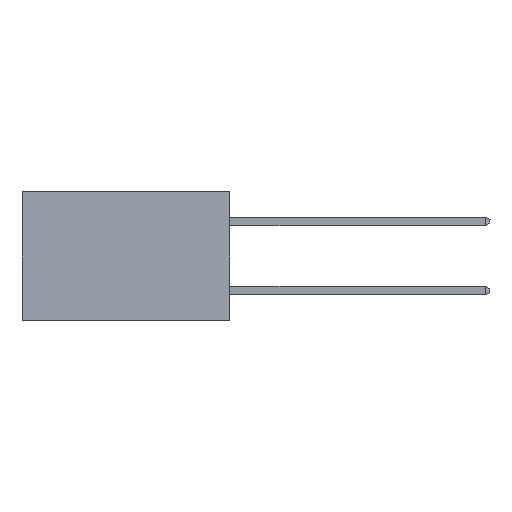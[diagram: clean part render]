
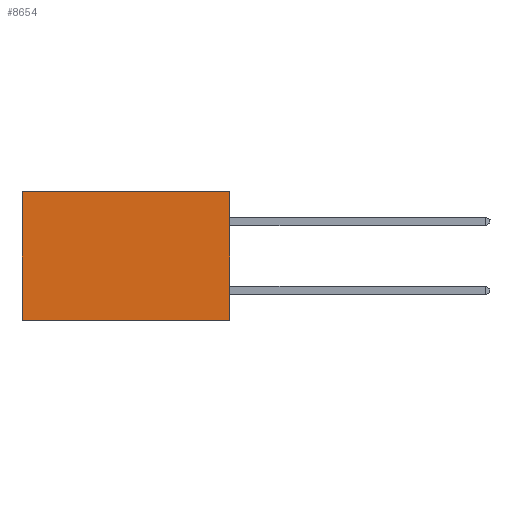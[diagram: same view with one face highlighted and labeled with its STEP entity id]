
A CAD part, left-side view. The second image highlights one B-rep face of the part: STEP entity #8654.
In plain terms, the highlighted planar face has unit normal (-1, 0, 0).
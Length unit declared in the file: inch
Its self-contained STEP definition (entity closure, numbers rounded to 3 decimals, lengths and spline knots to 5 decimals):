
#63 = EDGE_CURVE ( 'NONE', #13711, #1478, #19436, .T. ) ;
#925 = DIRECTION ( 'NONE',  ( 0., 0., -1. ) ) ;
#1478 = VERTEX_POINT ( 'NONE', #13507 ) ;
#2407 = DIRECTION ( 'NONE',  ( 0., 1., 0. ) ) ;
#2494 = ORIENTED_EDGE ( 'NONE', *, *, #6454, .F. ) ;
#3353 = VECTOR ( 'NONE', #8710, 39.37008 ) ;
#4126 = VECTOR ( 'NONE', #11520, 39.37008 ) ;
#4260 = VECTOR ( 'NONE', #9611, 39.37008 ) ;
#4748 = LINE ( 'NONE', #16527, #4126 ) ;
#5130 = VECTOR ( 'NONE', #2407, 39.37008 ) ;
#5297 = EDGE_CURVE ( 'NONE', #5812, #1478, #11095, .T. ) ;
#5747 = ORIENTED_EDGE ( 'NONE', *, *, #63, .T. ) ;
#5812 = VERTEX_POINT ( 'NONE', #21514 ) ;
#6288 = AXIS2_PLACEMENT_3D ( 'NONE', #6606, #20512, #925 ) ;
#6454 = EDGE_CURVE ( 'NONE', #19823, #5812, #20663, .T. ) ;
#6606 = CARTESIAN_POINT ( 'NONE',  ( 0.2615, 0., -0.37 ) ) ;
#7775 = CARTESIAN_POINT ( 'NONE',  ( 0.2615, 0.6, -0.37 ) ) ;
#8654 = ADVANCED_FACE ( 'NONE', ( #11764 ), #10047, .F. ) ;
#8710 = DIRECTION ( 'NONE',  ( 0., 0., -1. ) ) ;
#8977 = EDGE_CURVE ( 'NONE', #19823, #13711, #4748, .T. ) ;
#9542 = ORIENTED_EDGE ( 'NONE', *, *, #5297, .F. ) ;
#9611 = DIRECTION ( 'NONE',  ( 0., 0., -1. ) ) ;
#10047 = PLANE ( 'NONE',  #6288 ) ;
#11095 = LINE ( 'NONE', #18023, #5130 ) ;
#11520 = DIRECTION ( 'NONE',  ( 0., 1., 0. ) ) ;
#11546 = ORIENTED_EDGE ( 'NONE', *, *, #8977, .T. ) ;
#11764 = FACE_OUTER_BOUND ( 'NONE', #12062, .T. ) ;
#12062 = EDGE_LOOP ( 'NONE', ( #5747, #9542, #2494, #11546 ) ) ;
#13160 = CARTESIAN_POINT ( 'NONE',  ( 0.2615, 0., 0. ) ) ;
#13507 = CARTESIAN_POINT ( 'NONE',  ( 0.2615, 0.6, -0.37 ) ) ;
#13711 = VERTEX_POINT ( 'NONE', #15344 ) ;
#15344 = CARTESIAN_POINT ( 'NONE',  ( 0.2615, 0.6, 0. ) ) ;
#16527 = CARTESIAN_POINT ( 'NONE',  ( 0.2615, 0., 0. ) ) ;
#18023 = CARTESIAN_POINT ( 'NONE',  ( 0.2615, 0., -0.37 ) ) ;
#19436 = LINE ( 'NONE', #7775, #4260 ) ;
#19823 = VERTEX_POINT ( 'NONE', #13160 ) ;
#20512 = DIRECTION ( 'NONE',  ( 1., 0., 0. ) ) ;
#20663 = LINE ( 'NONE', #21121, #3353 ) ;
#21121 = CARTESIAN_POINT ( 'NONE',  ( 0.2615, 0., -0.37 ) ) ;
#21514 = CARTESIAN_POINT ( 'NONE',  ( 0.2615, 0., -0.37 ) ) ;
